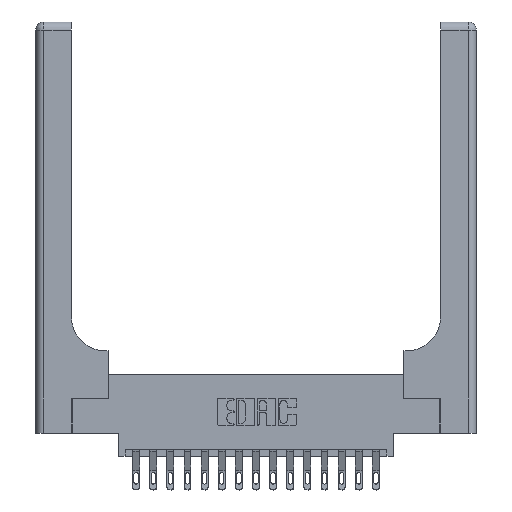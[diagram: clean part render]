
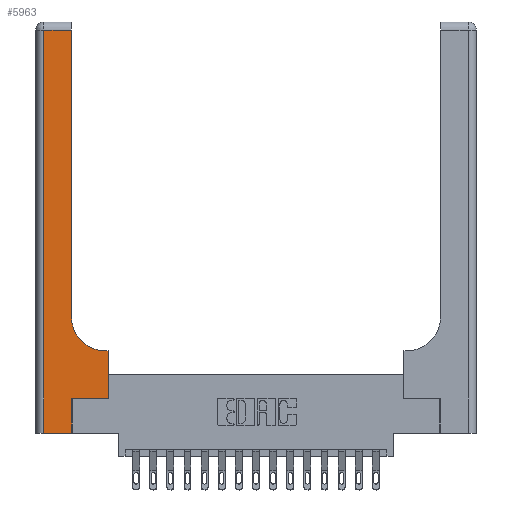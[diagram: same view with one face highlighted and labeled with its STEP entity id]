
A CAD part, top view. The second image highlights one B-rep face of the part: STEP entity #5963.
In plain terms, the highlighted planar face has unit normal (0, 0, 1).
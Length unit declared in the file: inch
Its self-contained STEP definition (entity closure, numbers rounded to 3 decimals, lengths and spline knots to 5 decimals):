
#24 = ORIENTED_EDGE ( 'NONE', *, *, #13500, .T. ) ;
#26 = CARTESIAN_POINT ( 'NONE',  ( 0.06, 3., 0.37 ) ) ;
#283 = CARTESIAN_POINT ( 'NONE',  ( 0.265, 0.25, 0.37 ) ) ;
#409 = CARTESIAN_POINT ( 'NONE',  ( 0.06, 2.94, 0.37 ) ) ;
#1057 = CARTESIAN_POINT ( 'NONE',  ( 0., 0., 0.37 ) ) ;
#1097 = VECTOR ( 'NONE', #6328, 39.37008 ) ;
#1496 = VECTOR ( 'NONE', #18006, 39.37008 ) ;
#1538 = VECTOR ( 'NONE', #13599, 39.37008 ) ;
#1747 = VECTOR ( 'NONE', #7065, 39.37008 ) ;
#1757 = ORIENTED_EDGE ( 'NONE', *, *, #3898, .T. ) ;
#1814 = EDGE_LOOP ( 'NONE', ( #5065, #14619, #5695, #12836, #1757, #24, #1817, #1947, #8778 ) ) ;
#1817 = ORIENTED_EDGE ( 'NONE', *, *, #11673, .T. ) ;
#1828 = FACE_OUTER_BOUND ( 'NONE', #1814, .T. ) ;
#1928 = CARTESIAN_POINT ( 'NONE',  ( 0.26, 3., 0.37 ) ) ;
#1947 = ORIENTED_EDGE ( 'NONE', *, *, #15541, .T. ) ;
#2249 = CARTESIAN_POINT ( 'NONE',  ( 0.528, 0.6, 0.37 ) ) ;
#2504 = CARTESIAN_POINT ( 'NONE',  ( 0.265, 0., 0.37 ) ) ;
#2961 = VECTOR ( 'NONE', #17085, 39.37008 ) ;
#3073 = VERTEX_POINT ( 'NONE', #16507 ) ;
#3523 = CARTESIAN_POINT ( 'NONE',  ( 0.26, 2.94, 0.37 ) ) ;
#3880 = CARTESIAN_POINT ( 'NONE',  ( 0.528, 0.25, 0.37 ) ) ;
#3898 = EDGE_CURVE ( 'NONE', #5269, #12363, #15083, .T. ) ;
#4341 = VERTEX_POINT ( 'NONE', #2249 ) ;
#4868 = LINE ( 'NONE', #12001, #1097 ) ;
#4881 = CARTESIAN_POINT ( 'NONE',  ( 0.51, 0.85, 0.37 ) ) ;
#4897 = DIRECTION ( 'NONE',  ( 0., 1., 0. ) ) ;
#5005 = VERTEX_POINT ( 'NONE', #409 ) ;
#5065 = ORIENTED_EDGE ( 'NONE', *, *, #15188, .T. ) ;
#5269 = VERTEX_POINT ( 'NONE', #2504 ) ;
#5537 = DIRECTION ( 'NONE',  ( 0., 1., 0. ) ) ;
#5695 = ORIENTED_EDGE ( 'NONE', *, *, #16964, .T. ) ;
#5865 = CARTESIAN_POINT ( 'NONE',  ( 0.26, 0.6, 0.37 ) ) ;
#5963 = ADVANCED_FACE ( 'NONE', ( #1828 ), #9221, .F. ) ;
#6029 = CARTESIAN_POINT ( 'NONE',  ( 0.528, 0.25, 0.37 ) ) ;
#6328 = DIRECTION ( 'NONE',  ( -1., 0., 0. ) ) ;
#6781 = VERTEX_POINT ( 'NONE', #10674 ) ;
#7065 = DIRECTION ( 'NONE',  ( 1., 0., 0. ) ) ;
#7381 = LINE ( 'NONE', #283, #2961 ) ;
#7582 = EDGE_CURVE ( 'NONE', #6781, #5269, #8550, .T. ) ;
#7756 = AXIS2_PLACEMENT_3D ( 'NONE', #4881, #18322, #14283 ) ;
#7839 = DIRECTION ( 'NONE',  ( 0., 0., -1. ) ) ;
#8257 = CARTESIAN_POINT ( 'NONE',  ( 0.265, 0.25, 0.37 ) ) ;
#8404 = LINE ( 'NONE', #3880, #10164 ) ;
#8550 = LINE ( 'NONE', #1057, #1747 ) ;
#8778 = ORIENTED_EDGE ( 'NONE', *, *, #16663, .T. ) ;
#9221 = PLANE ( 'NONE',  #17053 ) ;
#10164 = VECTOR ( 'NONE', #5537, 39.37008 ) ;
#10558 = VECTOR ( 'NONE', #4897, 39.37008 ) ;
#10578 = VECTOR ( 'NONE', #11914, 39.37008 ) ;
#10674 = CARTESIAN_POINT ( 'NONE',  ( 0.06, 0., 0.37 ) ) ;
#11021 = VERTEX_POINT ( 'NONE', #3523 ) ;
#11673 = EDGE_CURVE ( 'NONE', #16945, #4341, #8404, .T. ) ;
#11894 = CIRCLE ( 'NONE', #7756, 0.25 ) ;
#11914 = DIRECTION ( 'NONE',  ( -1., 0., 0. ) ) ;
#12001 = CARTESIAN_POINT ( 'NONE',  ( 0., 2.94, 0.37 ) ) ;
#12363 = VERTEX_POINT ( 'NONE', #8257 ) ;
#12836 = ORIENTED_EDGE ( 'NONE', *, *, #7582, .T. ) ;
#13500 = EDGE_CURVE ( 'NONE', #12363, #16945, #7381, .T. ) ;
#13599 = DIRECTION ( 'NONE',  ( 0., 1., 0. ) ) ;
#13813 = LINE ( 'NONE', #1928, #10558 ) ;
#13902 = DIRECTION ( 'NONE',  ( -1., 0., 0. ) ) ;
#14283 = DIRECTION ( 'NONE',  ( 1., 0., 0. ) ) ;
#14485 = EDGE_CURVE ( 'NONE', #11021, #5005, #4868, .T. ) ;
#14619 = ORIENTED_EDGE ( 'NONE', *, *, #14485, .T. ) ;
#14767 = LINE ( 'NONE', #26, #1496 ) ;
#15083 = LINE ( 'NONE', #15371, #1538 ) ;
#15188 = EDGE_CURVE ( 'NONE', #17456, #11021, #13813, .T. ) ;
#15271 = CARTESIAN_POINT ( 'NONE',  ( 0., 3., 0.37 ) ) ;
#15371 = CARTESIAN_POINT ( 'NONE',  ( 0.265, 0., 0.37 ) ) ;
#15541 = EDGE_CURVE ( 'NONE', #4341, #3073, #17733, .T. ) ;
#15867 = CARTESIAN_POINT ( 'NONE',  ( 0.26, 0.85, 0.37 ) ) ;
#16507 = CARTESIAN_POINT ( 'NONE',  ( 0.51, 0.6, 0.37 ) ) ;
#16663 = EDGE_CURVE ( 'NONE', #3073, #17456, #11894, .T. ) ;
#16945 = VERTEX_POINT ( 'NONE', #6029 ) ;
#16964 = EDGE_CURVE ( 'NONE', #5005, #6781, #14767, .T. ) ;
#17053 = AXIS2_PLACEMENT_3D ( 'NONE', #15271, #7839, #13902 ) ;
#17085 = DIRECTION ( 'NONE',  ( 1., 0., 0. ) ) ;
#17456 = VERTEX_POINT ( 'NONE', #15867 ) ;
#17733 = LINE ( 'NONE', #5865, #10578 ) ;
#18006 = DIRECTION ( 'NONE',  ( 0., -1., 0. ) ) ;
#18322 = DIRECTION ( 'NONE',  ( 0., 0., -1. ) ) ;
